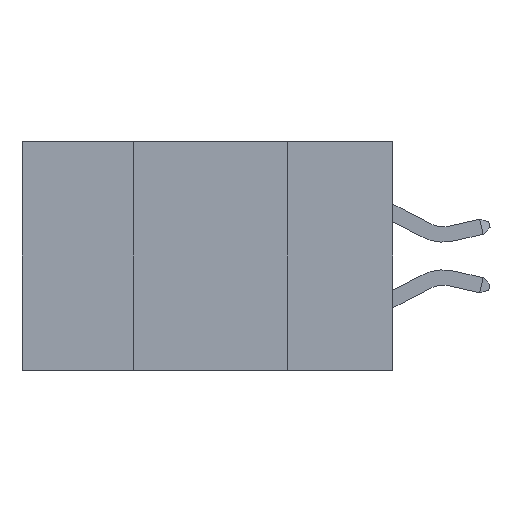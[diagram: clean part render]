
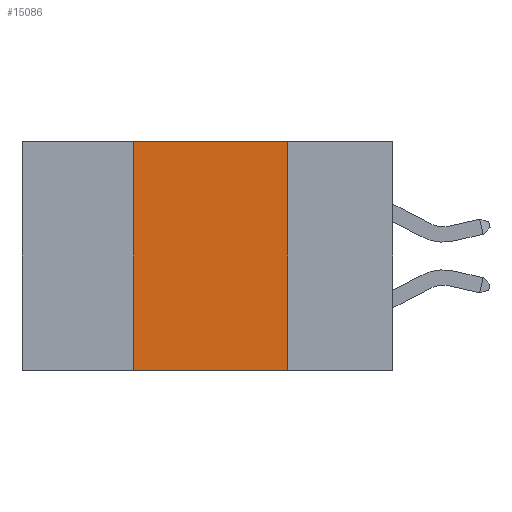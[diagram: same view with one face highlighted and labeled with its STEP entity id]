
A CAD part, left-side view. The second image highlights one B-rep face of the part: STEP entity #15086.
In plain terms, the highlighted planar face has unit normal (-1, 0, 0).
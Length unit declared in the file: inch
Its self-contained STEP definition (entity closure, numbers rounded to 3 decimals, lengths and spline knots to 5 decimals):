
#88 = DIRECTION ( 'NONE',  ( 0., 0., -1. ) ) ;
#949 = VERTEX_POINT ( 'NONE', #5404 ) ;
#1070 = LINE ( 'NONE', #5666, #7373 ) ;
#1654 = VECTOR ( 'NONE', #10275, 39.37008 ) ;
#2360 = VECTOR ( 'NONE', #11655, 39.37008 ) ;
#2746 = CARTESIAN_POINT ( 'NONE',  ( 0., 0.42, 0. ) ) ;
#2949 = FACE_OUTER_BOUND ( 'NONE', #6810, .T. ) ;
#3030 = EDGE_CURVE ( 'NONE', #949, #14528, #7950, .T. ) ;
#3034 = VERTEX_POINT ( 'NONE', #9990 ) ;
#3324 = EDGE_CURVE ( 'NONE', #14528, #3034, #1070, .T. ) ;
#3726 = ORIENTED_EDGE ( 'NONE', *, *, #4649, .T. ) ;
#4412 = DIRECTION ( 'NONE',  ( 0., 0., -1. ) ) ;
#4537 = CARTESIAN_POINT ( 'NONE',  ( 0., 0.6, 0. ) ) ;
#4649 = EDGE_CURVE ( 'NONE', #5214, #3034, #5503, .T. ) ;
#4821 = PLANE ( 'NONE',  #14251 ) ;
#5011 = DIRECTION ( 'NONE',  ( 0., 0., 1. ) ) ;
#5214 = VERTEX_POINT ( 'NONE', #8994 ) ;
#5404 = CARTESIAN_POINT ( 'NONE',  ( 0., 0.42, 0. ) ) ;
#5503 = LINE ( 'NONE', #14601, #2360 ) ;
#5666 = CARTESIAN_POINT ( 'NONE',  ( 0., 0.17, 0. ) ) ;
#6019 = CARTESIAN_POINT ( 'NONE',  ( 0., 0.6, 0. ) ) ;
#6568 = VECTOR ( 'NONE', #5011, 39.37008 ) ;
#6737 = EDGE_CURVE ( 'NONE', #5214, #949, #6932, .T. ) ;
#6810 = EDGE_LOOP ( 'NONE', ( #15120, #8818, #9572, #3726 ) ) ;
#6932 = LINE ( 'NONE', #2746, #6568 ) ;
#7212 = DIRECTION ( 'NONE',  ( 1., 0., 0. ) ) ;
#7373 = VECTOR ( 'NONE', #4412, 39.37008 ) ;
#7950 = LINE ( 'NONE', #4537, #1654 ) ;
#8818 = ORIENTED_EDGE ( 'NONE', *, *, #3030, .F. ) ;
#8994 = CARTESIAN_POINT ( 'NONE',  ( 0., 0.42, -0.37 ) ) ;
#9572 = ORIENTED_EDGE ( 'NONE', *, *, #6737, .F. ) ;
#9990 = CARTESIAN_POINT ( 'NONE',  ( 0., 0.17, -0.37 ) ) ;
#10275 = DIRECTION ( 'NONE',  ( 0., -1., 0. ) ) ;
#10695 = CARTESIAN_POINT ( 'NONE',  ( 0., 0.17, 0. ) ) ;
#11655 = DIRECTION ( 'NONE',  ( 0., -1., 0. ) ) ;
#14251 = AXIS2_PLACEMENT_3D ( 'NONE', #6019, #7212, #88 ) ;
#14528 = VERTEX_POINT ( 'NONE', #10695 ) ;
#14601 = CARTESIAN_POINT ( 'NONE',  ( 0., 0.6, -0.37 ) ) ;
#15086 = ADVANCED_FACE ( 'NONE', ( #2949 ), #4821, .F. ) ;
#15120 = ORIENTED_EDGE ( 'NONE', *, *, #3324, .F. ) ;
